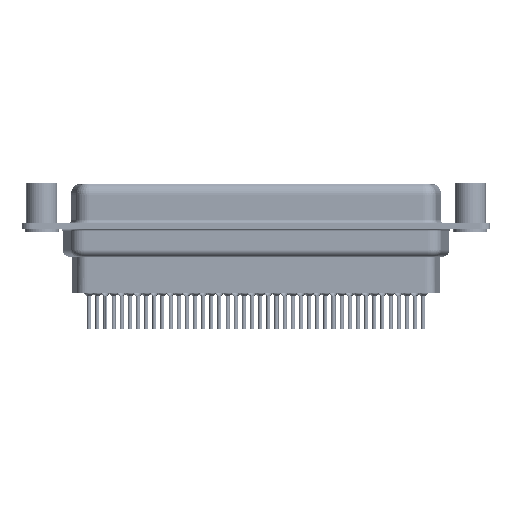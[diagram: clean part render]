
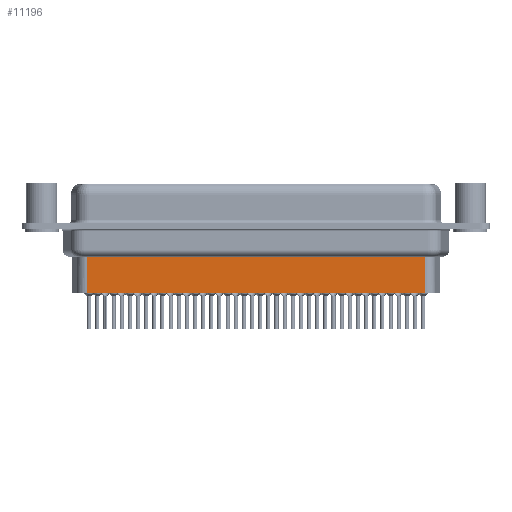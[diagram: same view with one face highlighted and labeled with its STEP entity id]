
A CAD part, front view. The second image highlights one B-rep face of the part: STEP entity #11196.
In plain terms, the highlighted planar face has unit normal (0, -1, 0).
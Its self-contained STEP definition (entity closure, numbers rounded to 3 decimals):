
#861 = LINE ( 'NONE', #15590, #31369 ) ;
#1689 = DIRECTION ( 'NONE',  ( -1., 0., 0. ) ) ;
#2024 = DIRECTION ( 'NONE',  ( 1., 0., 0. ) ) ;
#2474 = PLANE ( 'NONE',  #38123 ) ;
#5471 = CARTESIAN_POINT ( 'NONE',  ( 56.794, -3.5, -9.85 ) ) ;
#7409 = CARTESIAN_POINT ( 'NONE',  ( 6.706, -3.5, -9.85 ) ) ;
#7457 = DIRECTION ( 'NONE',  ( 0., 0., -1. ) ) ;
#7599 = VECTOR ( 'NONE', #29387, 1000. ) ;
#9300 = DIRECTION ( 'NONE',  ( 0., -1., 0. ) ) ;
#9683 = CARTESIAN_POINT ( 'NONE',  ( 6.459, -3.5, -4.097 ) ) ;
#10164 = ORIENTED_EDGE ( 'NONE', *, *, #10862, .T. ) ;
#10568 = VERTEX_POINT ( 'NONE', #14006 ) ;
#10862 = EDGE_CURVE ( 'NONE', #16246, #10568, #44178, .T. ) ;
#11196 = ADVANCED_FACE ( 'NONE', ( #24487 ), #2474, .T. ) ;
#11506 = VERTEX_POINT ( 'NONE', #23251 ) ;
#13629 = EDGE_CURVE ( 'NONE', #11506, #16837, #861, .T. ) ;
#14006 = CARTESIAN_POINT ( 'NONE',  ( 6.706, -3.5, -9.85 ) ) ;
#14908 = LINE ( 'NONE', #7409, #7599 ) ;
#15590 = CARTESIAN_POINT ( 'NONE',  ( 56.794, -3.5, -3.1 ) ) ;
#16246 = VERTEX_POINT ( 'NONE', #29309 ) ;
#16541 = CARTESIAN_POINT ( 'NONE',  ( 6.706, -3.5, -3.1 ) ) ;
#16593 = ORIENTED_EDGE ( 'NONE', *, *, #47143, .F. ) ;
#16837 = VERTEX_POINT ( 'NONE', #5471 ) ;
#18899 = ORIENTED_EDGE ( 'NONE', *, *, #40358, .T. ) ;
#20555 = LINE ( 'NONE', #9683, #44207 ) ;
#23251 = CARTESIAN_POINT ( 'NONE',  ( 56.794, -3.5, -4.097 ) ) ;
#24487 = FACE_OUTER_BOUND ( 'NONE', #33687, .T. ) ;
#25804 = CARTESIAN_POINT ( 'NONE',  ( 6.706, -3.5, -3.1 ) ) ;
#29309 = CARTESIAN_POINT ( 'NONE',  ( 6.706, -3.5, -4.097 ) ) ;
#29387 = DIRECTION ( 'NONE',  ( -1., 0., 0. ) ) ;
#30339 = DIRECTION ( 'NONE',  ( 0., 0., -1. ) ) ;
#31369 = VECTOR ( 'NONE', #30339, 1000. ) ;
#33687 = EDGE_LOOP ( 'NONE', ( #35683, #18899, #10164, #16593 ) ) ;
#35683 = ORIENTED_EDGE ( 'NONE', *, *, #13629, .F. ) ;
#38123 = AXIS2_PLACEMENT_3D ( 'NONE', #16541, #9300, #2024 ) ;
#40358 = EDGE_CURVE ( 'NONE', #11506, #16246, #20555, .T. ) ;
#41984 = VECTOR ( 'NONE', #7457, 1000. ) ;
#44178 = LINE ( 'NONE', #25804, #41984 ) ;
#44207 = VECTOR ( 'NONE', #1689, 1000. ) ;
#47143 = EDGE_CURVE ( 'NONE', #16837, #10568, #14908, .T. ) ;
